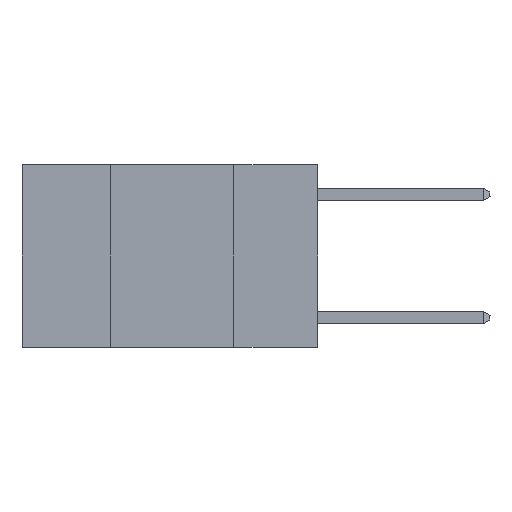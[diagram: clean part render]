
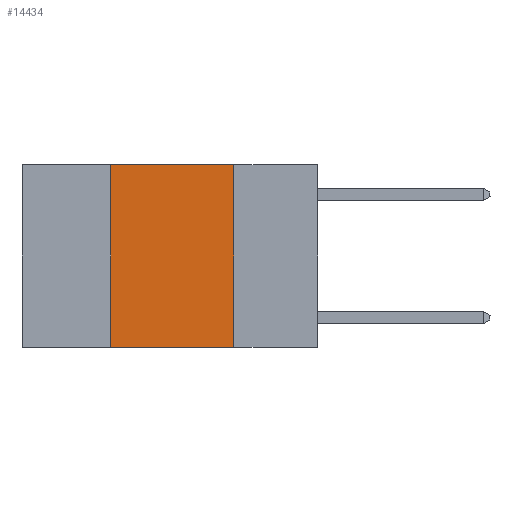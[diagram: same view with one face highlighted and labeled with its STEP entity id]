
A CAD part, left-side view. The second image highlights one B-rep face of the part: STEP entity #14434.
In plain terms, the highlighted planar face has unit normal (-1, 0, 0).
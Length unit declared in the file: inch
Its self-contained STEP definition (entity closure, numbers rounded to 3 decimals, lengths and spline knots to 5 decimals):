
#181 = CARTESIAN_POINT ( 'NONE',  ( 0., 0.42, -0.37 ) ) ;
#2226 = EDGE_CURVE ( 'NONE', #20893, #4889, #5175, .T. ) ;
#2965 = AXIS2_PLACEMENT_3D ( 'NONE', #12292, #3202, #16290 ) ;
#3202 = DIRECTION ( 'NONE',  ( 1., 0., 0. ) ) ;
#3351 = FACE_OUTER_BOUND ( 'NONE', #19318, .T. ) ;
#3413 = EDGE_CURVE ( 'NONE', #16613, #20893, #4448, .T. ) ;
#4334 = DIRECTION ( 'NONE',  ( 0., -1., 0. ) ) ;
#4448 = LINE ( 'NONE', #19880, #14026 ) ;
#4672 = VECTOR ( 'NONE', #26503, 39.37008 ) ;
#4889 = VERTEX_POINT ( 'NONE', #14407 ) ;
#5124 = PLANE ( 'NONE',  #2965 ) ;
#5175 = LINE ( 'NONE', #7223, #24069 ) ;
#7111 = CARTESIAN_POINT ( 'NONE',  ( 0., 0.6, -0.37 ) ) ;
#7223 = CARTESIAN_POINT ( 'NONE',  ( 0., 0.17, 0. ) ) ;
#11477 = VECTOR ( 'NONE', #4334, 39.37008 ) ;
#12292 = CARTESIAN_POINT ( 'NONE',  ( 0., 0.6, 0. ) ) ;
#12508 = ORIENTED_EDGE ( 'NONE', *, *, #2226, .F. ) ;
#13389 = DIRECTION ( 'NONE',  ( 0., -1., 0. ) ) ;
#14026 = VECTOR ( 'NONE', #13389, 39.37008 ) ;
#14407 = CARTESIAN_POINT ( 'NONE',  ( 0., 0.17, -0.37 ) ) ;
#14434 = ADVANCED_FACE ( 'NONE', ( #3351 ), #5124, .F. ) ;
#15186 = CARTESIAN_POINT ( 'NONE',  ( 0., 0.42, 0. ) ) ;
#16290 = DIRECTION ( 'NONE',  ( 0., 0., -1. ) ) ;
#16497 = EDGE_CURVE ( 'NONE', #20973, #4889, #24890, .T. ) ;
#16613 = VERTEX_POINT ( 'NONE', #18867 ) ;
#18867 = CARTESIAN_POINT ( 'NONE',  ( 0., 0.42, 0. ) ) ;
#19318 = EDGE_LOOP ( 'NONE', ( #12508, #27988, #24440, #28423 ) ) ;
#19880 = CARTESIAN_POINT ( 'NONE',  ( 0., 0.6, 0. ) ) ;
#20893 = VERTEX_POINT ( 'NONE', #21534 ) ;
#20973 = VERTEX_POINT ( 'NONE', #181 ) ;
#21534 = CARTESIAN_POINT ( 'NONE',  ( 0., 0.17, 0. ) ) ;
#21811 = LINE ( 'NONE', #15186, #4672 ) ;
#22099 = EDGE_CURVE ( 'NONE', #20973, #16613, #21811, .T. ) ;
#24069 = VECTOR ( 'NONE', #25435, 39.37008 ) ;
#24440 = ORIENTED_EDGE ( 'NONE', *, *, #22099, .F. ) ;
#24890 = LINE ( 'NONE', #7111, #11477 ) ;
#25435 = DIRECTION ( 'NONE',  ( 0., 0., -1. ) ) ;
#26503 = DIRECTION ( 'NONE',  ( 0., 0., 1. ) ) ;
#27988 = ORIENTED_EDGE ( 'NONE', *, *, #3413, .F. ) ;
#28423 = ORIENTED_EDGE ( 'NONE', *, *, #16497, .T. ) ;
